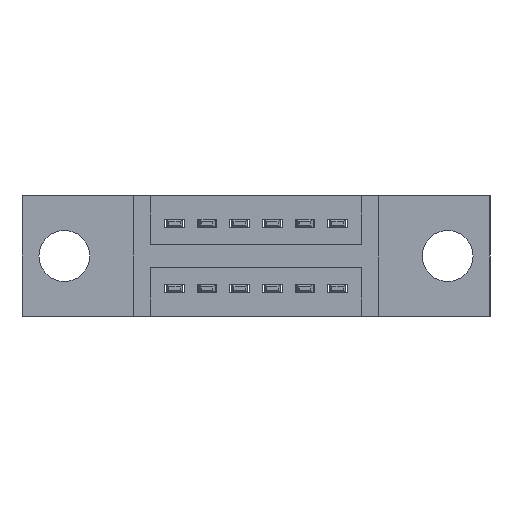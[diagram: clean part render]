
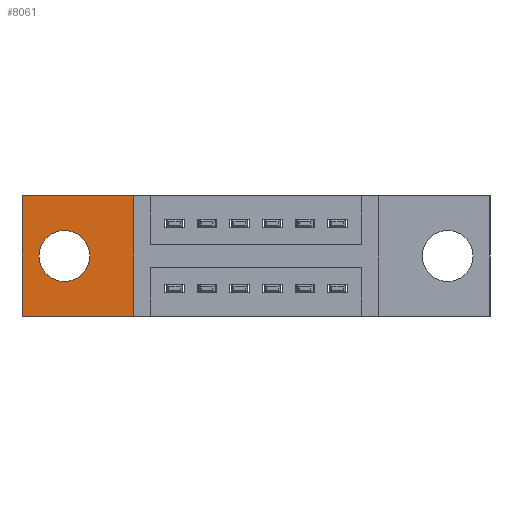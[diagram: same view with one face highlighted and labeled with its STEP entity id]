
A CAD part, front view. The second image highlights one B-rep face of the part: STEP entity #8061.
In plain terms, the highlighted planar face has unit normal (0, -1, 0).
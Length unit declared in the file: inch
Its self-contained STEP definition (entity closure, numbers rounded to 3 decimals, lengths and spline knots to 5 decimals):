
#131 = VECTOR ( 'NONE', #297, 39.37008 ) ;
#188 = CIRCLE ( 'NONE', #5848, 0.078 ) ;
#297 = DIRECTION ( 'NONE',  ( 0., 0., 1. ) ) ;
#576 = CARTESIAN_POINT ( 'NONE',  ( 0., 0.17, 0. ) ) ;
#634 = EDGE_CURVE ( 'NONE', #5884, #5642, #6203, .T. ) ;
#668 = CARTESIAN_POINT ( 'NONE',  ( 0., 0.17, -0.37 ) ) ;
#806 = DIRECTION ( 'NONE',  ( -1., 0., 0. ) ) ;
#972 = CARTESIAN_POINT ( 'NONE',  ( 0.13, 0.17, -0.263 ) ) ;
#993 = VECTOR ( 'NONE', #806, 39.37008 ) ;
#1135 = ORIENTED_EDGE ( 'NONE', *, *, #1550, .F. ) ;
#1232 = EDGE_CURVE ( 'NONE', #8908, #6339, #6955, .T. ) ;
#1482 = CARTESIAN_POINT ( 'NONE',  ( 0.13, 0.17, -0.107 ) ) ;
#1550 = EDGE_CURVE ( 'NONE', #6339, #8908, #188, .T. ) ;
#1612 = DIRECTION ( 'NONE',  ( 0., -1., 0. ) ) ;
#1636 = CARTESIAN_POINT ( 'NONE',  ( 0.3425, 0.17, 0. ) ) ;
#1662 = CARTESIAN_POINT ( 'NONE',  ( 0., 0.17, -0.37 ) ) ;
#1709 = DIRECTION ( 'NONE',  ( 0., 0., -1. ) ) ;
#1738 = VECTOR ( 'NONE', #7466, 39.37008 ) ;
#1965 = ORIENTED_EDGE ( 'NONE', *, *, #2559, .T. ) ;
#2316 = AXIS2_PLACEMENT_3D ( 'NONE', #4036, #4696, #8599 ) ;
#2416 = CARTESIAN_POINT ( 'NONE',  ( 0.3425, 0.17, -0.37 ) ) ;
#2559 = EDGE_CURVE ( 'NONE', #8120, #5908, #4401, .T. ) ;
#2787 = EDGE_CURVE ( 'NONE', #5908, #5884, #8601, .T. ) ;
#2907 = VECTOR ( 'NONE', #3015, 39.37008 ) ;
#2916 = AXIS2_PLACEMENT_3D ( 'NONE', #1662, #1612, #6850 ) ;
#3015 = DIRECTION ( 'NONE',  ( 0., 0., -1. ) ) ;
#4036 = CARTESIAN_POINT ( 'NONE',  ( 0.13, 0.17, -0.185 ) ) ;
#4401 = LINE ( 'NONE', #668, #1738 ) ;
#4524 = ORIENTED_EDGE ( 'NONE', *, *, #1232, .F. ) ;
#4696 = DIRECTION ( 'NONE',  ( 0., -1., 0. ) ) ;
#4786 = CARTESIAN_POINT ( 'NONE',  ( 0.3425, 0.17, 0. ) ) ;
#5222 = EDGE_LOOP ( 'NONE', ( #6648, #1965, #7711, #8333 ) ) ;
#5642 = VERTEX_POINT ( 'NONE', #5793 ) ;
#5793 = CARTESIAN_POINT ( 'NONE',  ( 0., 0.17, 0. ) ) ;
#5848 = AXIS2_PLACEMENT_3D ( 'NONE', #8756, #7140, #1709 ) ;
#5884 = VERTEX_POINT ( 'NONE', #1636 ) ;
#5908 = VERTEX_POINT ( 'NONE', #2416 ) ;
#6203 = LINE ( 'NONE', #7045, #993 ) ;
#6204 = PLANE ( 'NONE',  #2916 ) ;
#6339 = VERTEX_POINT ( 'NONE', #1482 ) ;
#6648 = ORIENTED_EDGE ( 'NONE', *, *, #8870, .T. ) ;
#6850 = DIRECTION ( 'NONE',  ( 0., 0., -1. ) ) ;
#6955 = CIRCLE ( 'NONE', #2316, 0.078 ) ;
#6998 = FACE_BOUND ( 'NONE', #9636, .T. ) ;
#7045 = CARTESIAN_POINT ( 'NONE',  ( 0., 0.17, 0. ) ) ;
#7095 = CARTESIAN_POINT ( 'NONE',  ( 0., 0.17, -0.37 ) ) ;
#7140 = DIRECTION ( 'NONE',  ( 0., -1., 0. ) ) ;
#7466 = DIRECTION ( 'NONE',  ( 1., 0., 0. ) ) ;
#7711 = ORIENTED_EDGE ( 'NONE', *, *, #2787, .T. ) ;
#8061 = ADVANCED_FACE ( 'NONE', ( #6998, #9339 ), #6204, .T. ) ;
#8120 = VERTEX_POINT ( 'NONE', #7095 ) ;
#8333 = ORIENTED_EDGE ( 'NONE', *, *, #634, .T. ) ;
#8599 = DIRECTION ( 'NONE',  ( 0., 0., -1. ) ) ;
#8601 = LINE ( 'NONE', #4786, #131 ) ;
#8756 = CARTESIAN_POINT ( 'NONE',  ( 0.13, 0.17, -0.185 ) ) ;
#8870 = EDGE_CURVE ( 'NONE', #5642, #8120, #9922, .T. ) ;
#8908 = VERTEX_POINT ( 'NONE', #972 ) ;
#9339 = FACE_OUTER_BOUND ( 'NONE', #5222, .T. ) ;
#9636 = EDGE_LOOP ( 'NONE', ( #1135, #4524 ) ) ;
#9922 = LINE ( 'NONE', #576, #2907 ) ;
